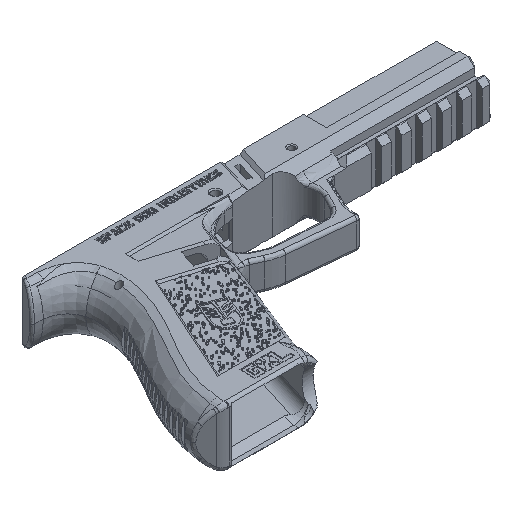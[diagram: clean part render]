
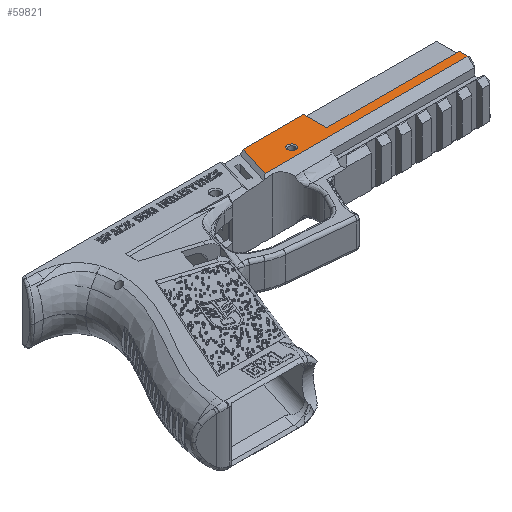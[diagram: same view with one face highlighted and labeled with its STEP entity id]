
A CAD part, isometric view. The second image highlights one B-rep face of the part: STEP entity #59821.
In plain terms, the highlighted planar face has unit normal (0, 0, 1).
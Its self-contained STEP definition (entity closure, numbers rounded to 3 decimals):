
#6484=CIRCLE('',#63452,2.025);
#6680=FACE_BOUND('',#11971,.T.);
#8356=FACE_OUTER_BOUND('',#11970,.T.);
#11970=EDGE_LOOP('',(#39769,#39770,#39771,#39772,#39773,#39774));
#11971=EDGE_LOOP('',(#39775));
#16016=LINE('',#71795,#20025);
#16022=LINE('',#71832,#20031);
#16031=LINE('',#71851,#20040);
#16032=LINE('',#71853,#20041);
#16033=LINE('',#71855,#20042);
#16034=LINE('',#71856,#20043);
#20025=VECTOR('',#64896,10.);
#20031=VECTOR('',#64906,10.);
#20040=VECTOR('',#64919,10.);
#20041=VECTOR('',#64920,10.);
#20042=VECTOR('',#64921,10.);
#20043=VECTOR('',#64922,10.);
#24034=VERTEX_POINT('',#71792);
#24035=VERTEX_POINT('',#71794);
#24043=VERTEX_POINT('',#71830);
#24051=VERTEX_POINT('',#71850);
#24052=VERTEX_POINT('',#71852);
#24053=VERTEX_POINT('',#71854);
#24054=VERTEX_POINT('',#71857);
#30291=EDGE_CURVE('',#24034,#24035,#16016,.T.);
#30301=EDGE_CURVE('',#24043,#24034,#16022,.T.);
#30310=EDGE_CURVE('',#24051,#24043,#16031,.T.);
#30311=EDGE_CURVE('',#24051,#24052,#16032,.T.);
#30312=EDGE_CURVE('',#24053,#24052,#16033,.T.);
#30313=EDGE_CURVE('',#24035,#24053,#16034,.T.);
#30314=EDGE_CURVE('',#24054,#24054,#6484,.T.);
#39769=ORIENTED_EDGE('',*,*,#30301,.F.);
#39770=ORIENTED_EDGE('',*,*,#30310,.F.);
#39771=ORIENTED_EDGE('',*,*,#30311,.T.);
#39772=ORIENTED_EDGE('',*,*,#30312,.F.);
#39773=ORIENTED_EDGE('',*,*,#30313,.F.);
#39774=ORIENTED_EDGE('',*,*,#30291,.F.);
#39775=ORIENTED_EDGE('',*,*,#30314,.T.);
#58663=PLANE('',#63451);
#59821=ADVANCED_FACE('',(#8356,#6680),#58663,.F.);
#63451=AXIS2_PLACEMENT_3D('',#71849,#64917,#64918);
#63452=AXIS2_PLACEMENT_3D('',#71858,#64923,#64924);
#64896=DIRECTION('',(0.301,0.954,0.));
#64906=DIRECTION('',(-1.,0.,0.));
#64917=DIRECTION('center_axis',(0.,0.,
-1.));
#64918=DIRECTION('ref_axis',(0.,1.,0.));
#64919=DIRECTION('',(0.,-1.,0.));
#64920=DIRECTION('',(-1.,0.,0.));
#64921=DIRECTION('',(0.,-1.,0.));
#64922=DIRECTION('',(1.,0.,0.));
#64923=DIRECTION('center_axis',(0.,0.,
-1.));
#64924=DIRECTION('ref_axis',(0.776,-0.63,0.));
#71792=CARTESIAN_POINT('',(77.608,-14.037,93.145));
#71794=CARTESIAN_POINT('',(82.591,1.767,93.145));
#71795=CARTESIAN_POINT('',(82.185,0.48,93.145));
#71830=CARTESIAN_POINT('',(178.385,-14.037,93.145));
#71832=CARTESIAN_POINT('',(64.237,-14.037,93.145));
#71849=CARTESIAN_POINT('Origin',(103.31,1.259,93.145));
#71850=CARTESIAN_POINT('',(178.385,-9.733,93.145));
#71851=CARTESIAN_POINT('',(178.385,-11.849,93.145));
#71852=CARTESIAN_POINT('',(112.635,-9.733,93.145));
#71853=CARTESIAN_POINT('',(105.549,-9.733,93.145));
#71854=CARTESIAN_POINT('',(112.635,1.767,93.145));
#71855=CARTESIAN_POINT('',(112.635,1.513,93.145));
#71856=CARTESIAN_POINT('',(33.317,1.767,93.145));
#71857=CARTESIAN_POINT('',(97.469,-9.398,93.145));
#71858=CARTESIAN_POINT('Origin',(95.444,-9.398,93.145));
